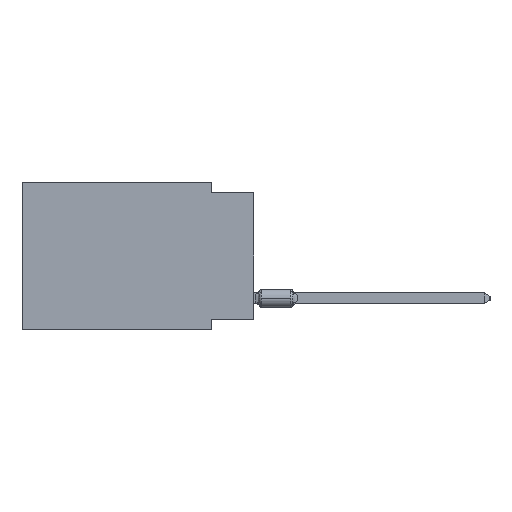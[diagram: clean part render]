
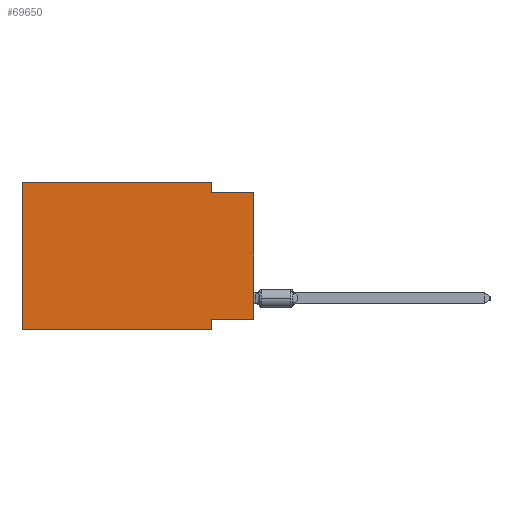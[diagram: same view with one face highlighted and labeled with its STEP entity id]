
A CAD part, left-side view. The second image highlights one B-rep face of the part: STEP entity #69650.
In plain terms, the highlighted planar face has unit normal (-1, 0, 0).
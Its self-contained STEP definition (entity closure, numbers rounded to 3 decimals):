
#375 = CARTESIAN_POINT ( 'NONE',  ( 0., 2.54, -8.255 ) ) ;
#932 = LINE ( 'NONE', #69487, #35469 ) ;
#4384 = VERTEX_POINT ( 'NONE', #12124 ) ;
#5607 = LINE ( 'NONE', #52921, #50080 ) ;
#6387 = VECTOR ( 'NONE', #13223, 1000. ) ;
#8754 = ORIENTED_EDGE ( 'NONE', *, *, #17195, .T. ) ;
#9427 = CARTESIAN_POINT ( 'NONE',  ( 0., 13.97, 0. ) ) ;
#9958 = VECTOR ( 'NONE', #65046, 1000. ) ;
#12124 = CARTESIAN_POINT ( 'NONE',  ( 0., 2.54, 0. ) ) ;
#12207 = DIRECTION ( 'NONE',  ( 0., -1., 0. ) ) ;
#12970 = VERTEX_POINT ( 'NONE', #26415 ) ;
#13223 = DIRECTION ( 'NONE',  ( 0., 0., 1. ) ) ;
#13713 = VERTEX_POINT ( 'NONE', #32425 ) ;
#15023 = ORIENTED_EDGE ( 'NONE', *, *, #50808, .F. ) ;
#15573 = VECTOR ( 'NONE', #51513, 1000. ) ;
#16887 = VERTEX_POINT ( 'NONE', #78684 ) ;
#17195 = EDGE_CURVE ( 'NONE', #13713, #16887, #85677, .T. ) ;
#18449 = DIRECTION ( 'NONE',  ( 0., 1., 0. ) ) ;
#23704 = ORIENTED_EDGE ( 'NONE', *, *, #87444, .F. ) ;
#26362 = VERTEX_POINT ( 'NONE', #40019 ) ;
#26415 = CARTESIAN_POINT ( 'NONE',  ( 0., 0., -8.255 ) ) ;
#27330 = VERTEX_POINT ( 'NONE', #375 ) ;
#28520 = DIRECTION ( 'NONE',  ( 0., 0., -1. ) ) ;
#29409 = VECTOR ( 'NONE', #85497, 1000. ) ;
#29413 = ORIENTED_EDGE ( 'NONE', *, *, #44263, .F. ) ;
#31068 = AXIS2_PLACEMENT_3D ( 'NONE', #75394, #68770, #28520 ) ;
#32425 = CARTESIAN_POINT ( 'NONE',  ( 0., 13.97, -8.89 ) ) ;
#32586 = DIRECTION ( 'NONE',  ( 0., -1., 0. ) ) ;
#35152 = FACE_OUTER_BOUND ( 'NONE', #54643, .T. ) ;
#35469 = VECTOR ( 'NONE', #81892, 1000. ) ;
#40019 = CARTESIAN_POINT ( 'NONE',  ( 0., 0., -0.635 ) ) ;
#41785 = PLANE ( 'NONE',  #31068 ) ;
#44263 = EDGE_CURVE ( 'NONE', #12970, #27330, #58292, .T. ) ;
#44524 = CARTESIAN_POINT ( 'NONE',  ( 0., 13.97, -8.89 ) ) ;
#44646 = ORIENTED_EDGE ( 'NONE', *, *, #51630, .T. ) ;
#45437 = CARTESIAN_POINT ( 'NONE',  ( 0., 0., -8.255 ) ) ;
#45763 = CARTESIAN_POINT ( 'NONE',  ( 0., 2.54, 0. ) ) ;
#50080 = VECTOR ( 'NONE', #32586, 1000. ) ;
#50808 = EDGE_CURVE ( 'NONE', #68315, #4384, #5607, .T. ) ;
#51513 = DIRECTION ( 'NONE',  ( 0., 0., -1. ) ) ;
#51630 = EDGE_CURVE ( 'NONE', #12970, #26362, #86689, .T. ) ;
#52921 = CARTESIAN_POINT ( 'NONE',  ( 0., 13.97, 0. ) ) ;
#53146 = LINE ( 'NONE', #80140, #29409 ) ;
#54643 = EDGE_LOOP ( 'NONE', ( #44646, #23704, #63770, #15023, #80841, #8754, #61461, #29413 ) ) ;
#55469 = LINE ( 'NONE', #9427, #9958 ) ;
#57915 = VERTEX_POINT ( 'NONE', #72903 ) ;
#58292 = LINE ( 'NONE', #45437, #86093 ) ;
#61461 = ORIENTED_EDGE ( 'NONE', *, *, #76623, .F. ) ;
#63770 = ORIENTED_EDGE ( 'NONE', *, *, #84703, .F. ) ;
#64814 = LINE ( 'NONE', #45763, #15573 ) ;
#65046 = DIRECTION ( 'NONE',  ( 0., 0., 1. ) ) ;
#65515 = CARTESIAN_POINT ( 'NONE',  ( 0., 13.97, 0. ) ) ;
#67178 = CARTESIAN_POINT ( 'NONE',  ( 0., 0., 0. ) ) ;
#68315 = VERTEX_POINT ( 'NONE', #65515 ) ;
#68770 = DIRECTION ( 'NONE',  ( 1., 0., 0. ) ) ;
#69487 = CARTESIAN_POINT ( 'NONE',  ( 0., 2.54, -8.89 ) ) ;
#69650 = ADVANCED_FACE ( 'NONE', ( #35152 ), #41785, .F. ) ;
#72903 = CARTESIAN_POINT ( 'NONE',  ( 0., 2.54, -0.635 ) ) ;
#75394 = CARTESIAN_POINT ( 'NONE',  ( 0., 13.97, 0. ) ) ;
#76623 = EDGE_CURVE ( 'NONE', #27330, #16887, #932, .T. ) ;
#78684 = CARTESIAN_POINT ( 'NONE',  ( 0., 2.54, -8.89 ) ) ;
#80140 = CARTESIAN_POINT ( 'NONE',  ( 0., 0., -0.635 ) ) ;
#80841 = ORIENTED_EDGE ( 'NONE', *, *, #84984, .F. ) ;
#81892 = DIRECTION ( 'NONE',  ( 0., 0., -1. ) ) ;
#83132 = VECTOR ( 'NONE', #12207, 1000. ) ;
#84703 = EDGE_CURVE ( 'NONE', #4384, #57915, #64814, .T. ) ;
#84984 = EDGE_CURVE ( 'NONE', #13713, #68315, #55469, .T. ) ;
#85497 = DIRECTION ( 'NONE',  ( 0., -1., 0. ) ) ;
#85677 = LINE ( 'NONE', #44524, #83132 ) ;
#86093 = VECTOR ( 'NONE', #18449, 1000. ) ;
#86689 = LINE ( 'NONE', #67178, #6387 ) ;
#87444 = EDGE_CURVE ( 'NONE', #57915, #26362, #53146, .T. ) ;
